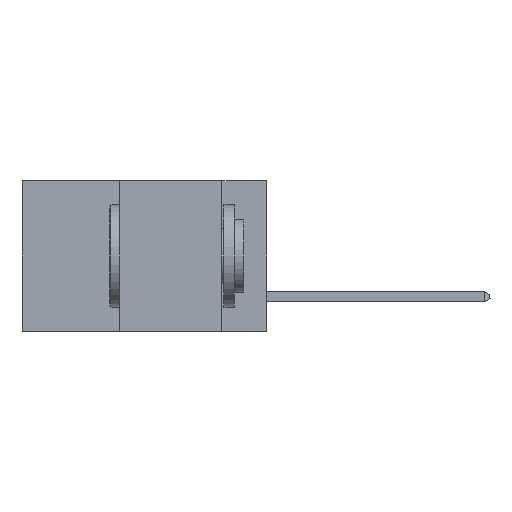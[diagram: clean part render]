
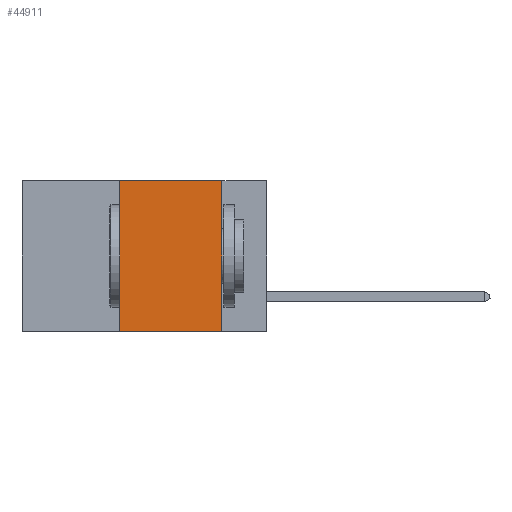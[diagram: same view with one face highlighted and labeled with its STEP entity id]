
A CAD part, left-side view. The second image highlights one B-rep face of the part: STEP entity #44911.
In plain terms, the highlighted planar face has unit normal (-1, 0, 0).
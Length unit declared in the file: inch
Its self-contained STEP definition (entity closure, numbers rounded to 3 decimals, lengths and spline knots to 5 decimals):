
#799 = DIRECTION ( 'NONE',  ( 0., 0., -1. ) ) ;
#946 = CARTESIAN_POINT ( 'NONE',  ( 0., 0.11, 0. ) ) ;
#1949 = VERTEX_POINT ( 'NONE', #16128 ) ;
#4994 = EDGE_CURVE ( 'NONE', #31933, #1949, #21158, .T. ) ;
#5521 = CARTESIAN_POINT ( 'NONE',  ( 0., 0.11, 0. ) ) ;
#6807 = ORIENTED_EDGE ( 'NONE', *, *, #14107, .T. ) ;
#7610 = VERTEX_POINT ( 'NONE', #946 ) ;
#9901 = CARTESIAN_POINT ( 'NONE',  ( 0., 0.36, -0.37 ) ) ;
#12593 = CARTESIAN_POINT ( 'NONE',  ( 0., 0.6, 0. ) ) ;
#12663 = DIRECTION ( 'NONE',  ( 0., 0., -1. ) ) ;
#14107 = EDGE_CURVE ( 'NONE', #31933, #38344, #37886, .T. ) ;
#16053 = DIRECTION ( 'NONE',  ( 1., 0., 0. ) ) ;
#16128 = CARTESIAN_POINT ( 'NONE',  ( 0., 0.36, 0. ) ) ;
#17735 = EDGE_LOOP ( 'NONE', ( #48273, #39039, #44109, #6807 ) ) ;
#19693 = CARTESIAN_POINT ( 'NONE',  ( 0., 0.6, 0. ) ) ;
#20283 = EDGE_CURVE ( 'NONE', #1949, #7610, #26202, .T. ) ;
#21158 = LINE ( 'NONE', #33007, #36579 ) ;
#23170 = PLANE ( 'NONE',  #29247 ) ;
#23690 = DIRECTION ( 'NONE',  ( 0., 0., 1. ) ) ;
#25786 = VECTOR ( 'NONE', #12663, 39.37008 ) ;
#26131 = CARTESIAN_POINT ( 'NONE',  ( 0., 0.6, -0.37 ) ) ;
#26202 = LINE ( 'NONE', #19693, #47629 ) ;
#26282 = FACE_OUTER_BOUND ( 'NONE', #17735, .T. ) ;
#27796 = VECTOR ( 'NONE', #48541, 39.37008 ) ;
#29247 = AXIS2_PLACEMENT_3D ( 'NONE', #12593, #16053, #799 ) ;
#31933 = VERTEX_POINT ( 'NONE', #9901 ) ;
#33007 = CARTESIAN_POINT ( 'NONE',  ( 0., 0.36, 0. ) ) ;
#36579 = VECTOR ( 'NONE', #23690, 39.37008 ) ;
#37766 = CARTESIAN_POINT ( 'NONE',  ( 0., 0.11, -0.37 ) ) ;
#37886 = LINE ( 'NONE', #26131, #27796 ) ;
#38344 = VERTEX_POINT ( 'NONE', #37766 ) ;
#39039 = ORIENTED_EDGE ( 'NONE', *, *, #20283, .F. ) ;
#39082 = EDGE_CURVE ( 'NONE', #7610, #38344, #44187, .T. ) ;
#44109 = ORIENTED_EDGE ( 'NONE', *, *, #4994, .F. ) ;
#44187 = LINE ( 'NONE', #5521, #25786 ) ;
#44911 = ADVANCED_FACE ( 'NONE', ( #26282 ), #23170, .F. ) ;
#45704 = DIRECTION ( 'NONE',  ( 0., -1., 0. ) ) ;
#47629 = VECTOR ( 'NONE', #45704, 39.37008 ) ;
#48273 = ORIENTED_EDGE ( 'NONE', *, *, #39082, .F. ) ;
#48541 = DIRECTION ( 'NONE',  ( 0., -1., 0. ) ) ;
